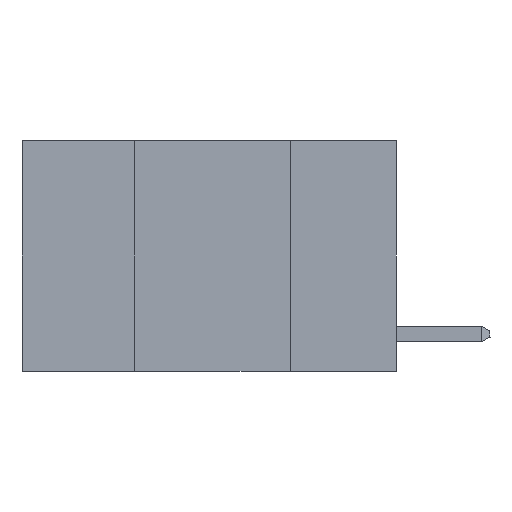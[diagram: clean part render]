
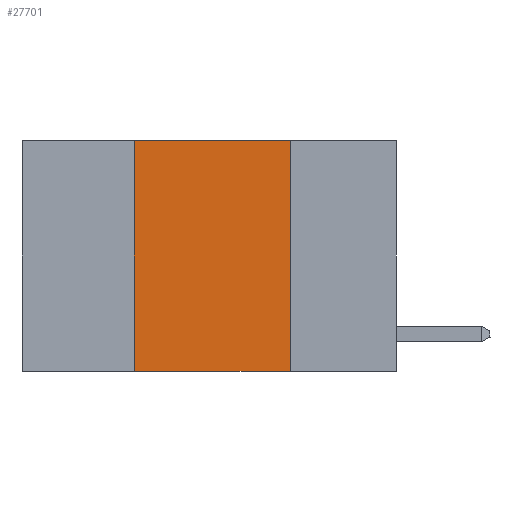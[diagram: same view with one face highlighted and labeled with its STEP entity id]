
A CAD part, left-side view. The second image highlights one B-rep face of the part: STEP entity #27701.
In plain terms, the highlighted planar face has unit normal (-1, 0, 0).
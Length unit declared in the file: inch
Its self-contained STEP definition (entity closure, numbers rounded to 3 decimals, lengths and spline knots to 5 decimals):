
#356 = DIRECTION ( 'NONE',  ( 0., 0., -1. ) ) ;
#2273 = ORIENTED_EDGE ( 'NONE', *, *, #28551, .F. ) ;
#4686 = CARTESIAN_POINT ( 'NONE',  ( 0., 0.42, 0. ) ) ;
#5369 = CARTESIAN_POINT ( 'NONE',  ( 0., 0.6, -0.37 ) ) ;
#5449 = CARTESIAN_POINT ( 'NONE',  ( 0., 0.6, 0. ) ) ;
#6629 = EDGE_CURVE ( 'NONE', #22915, #19892, #18183, .T. ) ;
#6676 = DIRECTION ( 'NONE',  ( 0., 0., 1. ) ) ;
#7526 = CARTESIAN_POINT ( 'NONE',  ( 0., 0.6, 0. ) ) ;
#7640 = DIRECTION ( 'NONE',  ( 0., -1., 0. ) ) ;
#7707 = AXIS2_PLACEMENT_3D ( 'NONE', #5449, #21152, #7824 ) ;
#7720 = PLANE ( 'NONE',  #7707 ) ;
#7824 = DIRECTION ( 'NONE',  ( 0., 0., -1. ) ) ;
#8855 = VERTEX_POINT ( 'NONE', #28673 ) ;
#9504 = ORIENTED_EDGE ( 'NONE', *, *, #10529, .F. ) ;
#9581 = VECTOR ( 'NONE', #6676, 39.37008 ) ;
#9766 = DIRECTION ( 'NONE',  ( 0., -1., 0. ) ) ;
#10529 = EDGE_CURVE ( 'NONE', #19892, #8855, #12640, .T. ) ;
#11515 = VECTOR ( 'NONE', #9766, 39.37008 ) ;
#11759 = ORIENTED_EDGE ( 'NONE', *, *, #15183, .T. ) ;
#12640 = LINE ( 'NONE', #27065, #23789 ) ;
#14880 = FACE_OUTER_BOUND ( 'NONE', #19696, .T. ) ;
#15183 = EDGE_CURVE ( 'NONE', #25685, #8855, #21731, .T. ) ;
#15522 = LINE ( 'NONE', #22279, #9581 ) ;
#18183 = LINE ( 'NONE', #7526, #11515 ) ;
#18549 = CARTESIAN_POINT ( 'NONE',  ( 0., 0.42, -0.37 ) ) ;
#19211 = ORIENTED_EDGE ( 'NONE', *, *, #6629, .F. ) ;
#19696 = EDGE_LOOP ( 'NONE', ( #9504, #19211, #2273, #11759 ) ) ;
#19892 = VERTEX_POINT ( 'NONE', #23066 ) ;
#21152 = DIRECTION ( 'NONE',  ( 1., 0., 0. ) ) ;
#21731 = LINE ( 'NONE', #5369, #26237 ) ;
#22279 = CARTESIAN_POINT ( 'NONE',  ( 0., 0.42, 0. ) ) ;
#22915 = VERTEX_POINT ( 'NONE', #4686 ) ;
#23066 = CARTESIAN_POINT ( 'NONE',  ( 0., 0.17, 0. ) ) ;
#23789 = VECTOR ( 'NONE', #356, 39.37008 ) ;
#25685 = VERTEX_POINT ( 'NONE', #18549 ) ;
#26237 = VECTOR ( 'NONE', #7640, 39.37008 ) ;
#27065 = CARTESIAN_POINT ( 'NONE',  ( 0., 0.17, 0. ) ) ;
#27701 = ADVANCED_FACE ( 'NONE', ( #14880 ), #7720, .F. ) ;
#28551 = EDGE_CURVE ( 'NONE', #25685, #22915, #15522, .T. ) ;
#28673 = CARTESIAN_POINT ( 'NONE',  ( 0., 0.17, -0.37 ) ) ;
